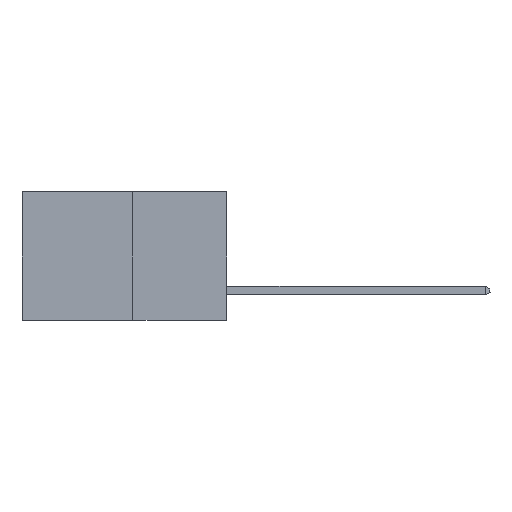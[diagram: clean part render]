
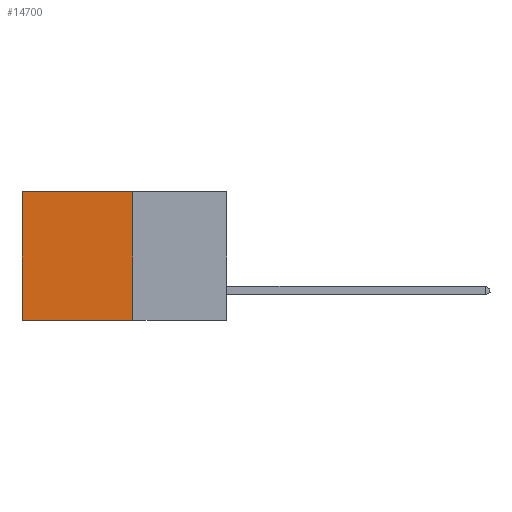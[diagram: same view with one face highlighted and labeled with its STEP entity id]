
A CAD part, left-side view. The second image highlights one B-rep face of the part: STEP entity #14700.
In plain terms, the highlighted planar face has unit normal (-1, 0, 0).
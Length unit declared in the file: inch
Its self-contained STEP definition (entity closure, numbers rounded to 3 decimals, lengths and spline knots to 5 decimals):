
#116 = EDGE_CURVE ( 'NONE', #23126, #27211, #16095, .T. ) ;
#892 = DIRECTION ( 'NONE',  ( 0., 0., -1. ) ) ;
#2219 = CARTESIAN_POINT ( 'NONE',  ( 0.277, 0.27, -0.37 ) ) ;
#5182 = EDGE_CURVE ( 'NONE', #12680, #23126, #13019, .T. ) ;
#6132 = DIRECTION ( 'NONE',  ( 1., 0., 0. ) ) ;
#7423 = VECTOR ( 'NONE', #25556, 39.37008 ) ;
#7439 = ORIENTED_EDGE ( 'NONE', *, *, #30719, .T. ) ;
#9112 = CARTESIAN_POINT ( 'NONE',  ( 0.277, 0.59, 0. ) ) ;
#12680 = VERTEX_POINT ( 'NONE', #24951 ) ;
#13019 = LINE ( 'NONE', #2219, #26795 ) ;
#14105 = ORIENTED_EDGE ( 'NONE', *, *, #5182, .F. ) ;
#14198 = VERTEX_POINT ( 'NONE', #9112 ) ;
#14700 = ADVANCED_FACE ( 'NONE', ( #18749 ), #16497, .F. ) ;
#14769 = DIRECTION ( 'NONE',  ( 0., 1., 0. ) ) ;
#15454 = EDGE_CURVE ( 'NONE', #14198, #27211, #27171, .T. ) ;
#15809 = CARTESIAN_POINT ( 'NONE',  ( 0.277, 0.59, -0.37 ) ) ;
#16095 = LINE ( 'NONE', #16223, #21417 ) ;
#16223 = CARTESIAN_POINT ( 'NONE',  ( 0.277, 0.27, -0.37 ) ) ;
#16497 = PLANE ( 'NONE',  #19536 ) ;
#16847 = EDGE_LOOP ( 'NONE', ( #24105, #32007, #14105, #7439 ) ) ;
#16922 = CARTESIAN_POINT ( 'NONE',  ( 0.277, 0.59, -0.37 ) ) ;
#17851 = CARTESIAN_POINT ( 'NONE',  ( 0.277, 0.27, 0. ) ) ;
#18749 = FACE_OUTER_BOUND ( 'NONE', #16847, .T. ) ;
#19536 = AXIS2_PLACEMENT_3D ( 'NONE', #21762, #6132, #24344 ) ;
#20246 = CARTESIAN_POINT ( 'NONE',  ( 0.277, 0.27, -0.37 ) ) ;
#21306 = LINE ( 'NONE', #17851, #7423 ) ;
#21417 = VECTOR ( 'NONE', #14769, 39.37008 ) ;
#21762 = CARTESIAN_POINT ( 'NONE',  ( 0.277, 0.27, -0.37 ) ) ;
#23126 = VERTEX_POINT ( 'NONE', #20246 ) ;
#24105 = ORIENTED_EDGE ( 'NONE', *, *, #15454, .T. ) ;
#24344 = DIRECTION ( 'NONE',  ( 0., 0., -1. ) ) ;
#24762 = DIRECTION ( 'NONE',  ( 0., 0., -1. ) ) ;
#24951 = CARTESIAN_POINT ( 'NONE',  ( 0.277, 0.27, 0. ) ) ;
#25556 = DIRECTION ( 'NONE',  ( 0., 1., 0. ) ) ;
#25568 = VECTOR ( 'NONE', #24762, 39.37008 ) ;
#26795 = VECTOR ( 'NONE', #892, 39.37008 ) ;
#27171 = LINE ( 'NONE', #16922, #25568 ) ;
#27211 = VERTEX_POINT ( 'NONE', #15809 ) ;
#30719 = EDGE_CURVE ( 'NONE', #12680, #14198, #21306, .T. ) ;
#32007 = ORIENTED_EDGE ( 'NONE', *, *, #116, .F. ) ;
